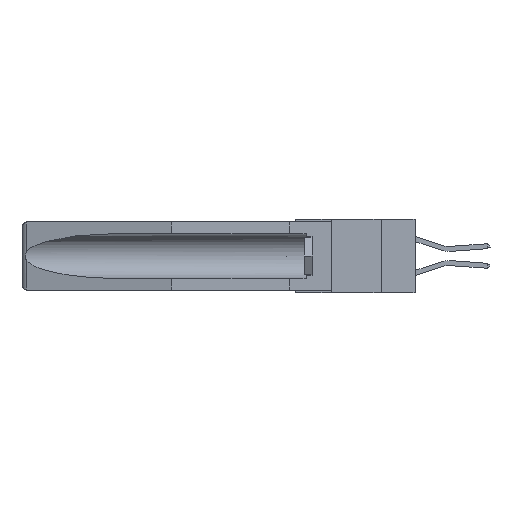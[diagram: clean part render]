
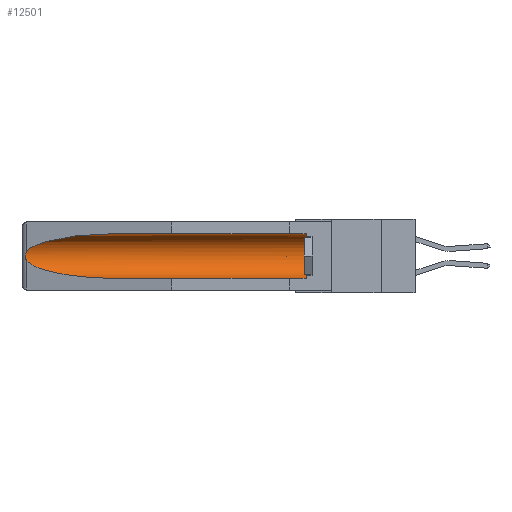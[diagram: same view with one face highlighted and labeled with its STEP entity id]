
A CAD part, left-side view. The second image highlights one B-rep face of the part: STEP entity #12501.
In plain terms, the highlighted cylindrical face has radius 2.857 mm (diameter 5.715 mm), a partial arc.
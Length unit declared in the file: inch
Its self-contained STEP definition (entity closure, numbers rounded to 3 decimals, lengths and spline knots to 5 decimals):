
#414 = ORIENTED_EDGE ( 'NONE', *, *, #9243, .F. ) ;
#472 = CARTESIAN_POINT ( 'NONE',  ( 0.155, 1.07973, -0.059 ) ) ;
#505 = EDGE_CURVE ( 'NONE', #26473, #33465, #769, .T. ) ;
#769 =( BOUNDED_CURVE ( )  B_SPLINE_CURVE ( 3, ( #21229, #29533, #15940, #35057 ),
 .UNSPECIFIED., .F., .F. ) 
 B_SPLINE_CURVE_WITH_KNOTS ( ( 4, 4 ),
 ( 4.71239, 6.08839 ),
 .UNSPECIFIED. ) 
 CURVE ( )  GEOMETRIC_REPRESENTATION_ITEM ( )  RATIONAL_B_SPLINE_CURVE ( ( 1., 0.848, 0.848, 1. ) ) 
 REPRESENTATION_ITEM ( '' )  );
#1263 = DIRECTION ( 'NONE',  ( 0., 0., 1. ) ) ;
#1272 = CARTESIAN_POINT ( 'NONE',  ( 0.2673, 1.5327, -0.16383 ) ) ;
#1396 =( BOUNDED_CURVE ( )  B_SPLINE_CURVE ( 3, ( #28371, #34367, #6953, #17786 ),
 .UNSPECIFIED., .F., .F. ) 
 B_SPLINE_CURVE_WITH_KNOTS ( ( 4, 4 ),
 ( 0.1948, 1.5708 ),
 .UNSPECIFIED. ) 
 CURVE ( )  GEOMETRIC_REPRESENTATION_ITEM ( )  RATIONAL_B_SPLINE_CURVE ( ( 1., 0.848, 0.848, 1. ) ) 
 REPRESENTATION_ITEM ( '' )  );
#1483 = EDGE_CURVE ( 'NONE', #11089, #11602, #14225, .T. ) ;
#1504 = CARTESIAN_POINT ( 'NONE',  ( 0.26654, 1.53092, -0.15636 ) ) ;
#1701 = EDGE_CURVE ( 'NONE', #33465, #20517, #28645, .T. ) ;
#1728 = CARTESIAN_POINT ( 'NONE',  ( 0.2675, 1.53308, -0.16763 ) ) ;
#2929 = CARTESIAN_POINT ( 'NONE',  ( 0.155, 0.126, -0.1715 ) ) ;
#3565 = LINE ( 'NONE', #33931, #30815 ) ;
#4111 = CARTESIAN_POINT ( 'NONE',  ( 0.26597, 1.52961, -0.15275 ) ) ;
#6726 = CARTESIAN_POINT ( 'NONE',  ( 0.26537, 1.52718, -0.19328 ) ) ;
#6910 = CARTESIAN_POINT ( 'NONE',  ( 0.155, 0.126, -0.059 ) ) ;
#6953 = CARTESIAN_POINT ( 'NONE',  ( 0.21114, 1.30732, -0.284 ) ) ;
#7711 = FACE_OUTER_BOUND ( 'NONE', #17842, .T. ) ;
#8100 = EDGE_CURVE ( 'NONE', #20517, #31729, #1396, .T. ) ;
#8455 = ORIENTED_EDGE ( 'NONE', *, *, #8100, .T. ) ;
#8511 = CARTESIAN_POINT ( 'NONE',  ( 0.155, 1.07973, -0.284 ) ) ;
#9243 = EDGE_CURVE ( 'NONE', #11089, #31729, #3565, .T. ) ;
#9734 = EDGE_CURVE ( 'NONE', #11602, #26473, #21394, .T. ) ;
#10644 = CARTESIAN_POINT ( 'NONE',  ( 0.155, 0.126, -0.284 ) ) ;
#11089 = VERTEX_POINT ( 'NONE', #10644 ) ;
#11602 = VERTEX_POINT ( 'NONE', #6910 ) ;
#12070 = AXIS2_PLACEMENT_3D ( 'NONE', #20193, #12422, #1263 ) ;
#12327 = CARTESIAN_POINT ( 'NONE',  ( 0.155, -0.30754, -0.059 ) ) ;
#12422 = DIRECTION ( 'NONE',  ( 0., 1., 0. ) ) ;
#12432 = CARTESIAN_POINT ( 'NONE',  ( 0.26537, 1.52718, -0.14972 ) ) ;
#12501 = ADVANCED_FACE ( 'NONE', ( #7711 ), #28573, .F. ) ;
#13313 = VECTOR ( 'NONE', #28488, 39.37008 ) ;
#13990 = DIRECTION ( 'NONE',  ( 0., -1., 0. ) ) ;
#14225 = CIRCLE ( 'NONE', #16105, 0.1125 ) ;
#14903 = CARTESIAN_POINT ( 'NONE',  ( 0.26597, 1.5296, -0.19026 ) ) ;
#15940 = CARTESIAN_POINT ( 'NONE',  ( 0.25451, 1.48313, -0.09465 ) ) ;
#16105 = AXIS2_PLACEMENT_3D ( 'NONE', #2929, #13990, #27438 ) ;
#17786 = CARTESIAN_POINT ( 'NONE',  ( 0.155, 1.07973, -0.284 ) ) ;
#17842 = EDGE_LOOP ( 'NONE', ( #29136, #27442, #8455, #414, #22929, #33655 ) ) ;
#20193 = CARTESIAN_POINT ( 'NONE',  ( 0.155, -0.30754, -0.1715 ) ) ;
#20517 = VERTEX_POINT ( 'NONE', #20825 ) ;
#20825 = CARTESIAN_POINT ( 'NONE',  ( 0.26537, 1.52718, -0.19328 ) ) ;
#21229 = CARTESIAN_POINT ( 'NONE',  ( 0.155, 1.07973, -0.059 ) ) ;
#21394 = LINE ( 'NONE', #12327, #13313 ) ;
#22929 = ORIENTED_EDGE ( 'NONE', *, *, #1483, .T. ) ;
#23242 = CARTESIAN_POINT ( 'NONE',  ( 0.26655, 1.53094, -0.18657 ) ) ;
#26473 = VERTEX_POINT ( 'NONE', #472 ) ;
#27438 = DIRECTION ( 'NONE',  ( 0., 0., 1. ) ) ;
#27442 = ORIENTED_EDGE ( 'NONE', *, *, #1701, .T. ) ;
#28371 = CARTESIAN_POINT ( 'NONE',  ( 0.26537, 1.52718, -0.19328 ) ) ;
#28488 = DIRECTION ( 'NONE',  ( 0., 1., 0. ) ) ;
#28573 = CYLINDRICAL_SURFACE ( 'NONE', #12070, 0.1125 ) ;
#28645 = B_SPLINE_CURVE_WITH_KNOTS ( 'NONE', 3,
 ( #12432, #4111, #1504, #1272, #1728, #28719, #31115, #23242, #14903, #6726 ),
 .UNSPECIFIED., .F., .F.,
 ( 4, 2, 2, 2, 4 ),
 ( 0., 0.00029, 0.00058, 0.00087, 0.00117 ),
 .UNSPECIFIED. ) ;
#28719 = CARTESIAN_POINT ( 'NONE',  ( 0.2675, 1.53308, -0.17534 ) ) ;
#29136 = ORIENTED_EDGE ( 'NONE', *, *, #505, .T. ) ;
#29533 = CARTESIAN_POINT ( 'NONE',  ( 0.21114, 1.30732, -0.059 ) ) ;
#29967 = CARTESIAN_POINT ( 'NONE',  ( 0.26537, 1.52718, -0.14972 ) ) ;
#30815 = VECTOR ( 'NONE', #34158, 39.37008 ) ;
#31115 = CARTESIAN_POINT ( 'NONE',  ( 0.2673, 1.53269, -0.17917 ) ) ;
#31729 = VERTEX_POINT ( 'NONE', #8511 ) ;
#33465 = VERTEX_POINT ( 'NONE', #29967 ) ;
#33655 = ORIENTED_EDGE ( 'NONE', *, *, #9734, .T. ) ;
#33931 = CARTESIAN_POINT ( 'NONE',  ( 0.155, -0.30754, -0.284 ) ) ;
#34158 = DIRECTION ( 'NONE',  ( 0., 1., 0. ) ) ;
#34367 = CARTESIAN_POINT ( 'NONE',  ( 0.25451, 1.48313, -0.24835 ) ) ;
#35057 = CARTESIAN_POINT ( 'NONE',  ( 0.26537, 1.52718, -0.14972 ) ) ;
